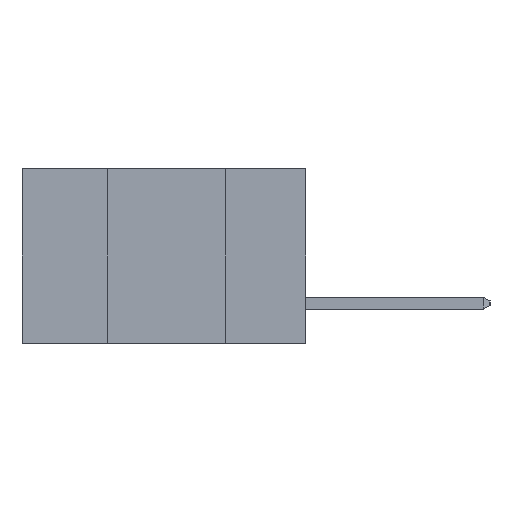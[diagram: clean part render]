
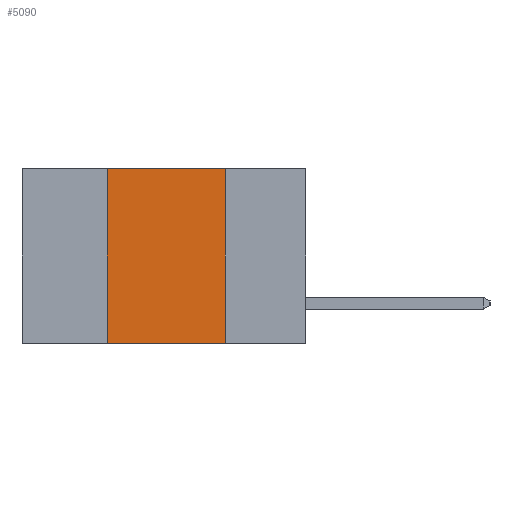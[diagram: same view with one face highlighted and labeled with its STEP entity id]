
A CAD part, left-side view. The second image highlights one B-rep face of the part: STEP entity #5090.
In plain terms, the highlighted planar face has unit normal (-1, 0, 0).
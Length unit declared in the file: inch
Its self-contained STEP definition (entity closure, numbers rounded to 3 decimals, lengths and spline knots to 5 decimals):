
#30 = EDGE_CURVE ( 'NONE', #3583, #1709, #10387, .T. ) ;
#32 = DIRECTION ( 'NONE',  ( 0., -1., 0. ) ) ;
#1709 = VERTEX_POINT ( 'NONE', #10174 ) ;
#1908 = EDGE_CURVE ( 'NONE', #9272, #1709, #5114, .T. ) ;
#2156 = DIRECTION ( 'NONE',  ( 0., 0., -1. ) ) ;
#2189 = ORIENTED_EDGE ( 'NONE', *, *, #1908, .T. ) ;
#2211 = VECTOR ( 'NONE', #10331, 39.37008 ) ;
#2306 = DIRECTION ( 'NONE',  ( 0., 0., -1. ) ) ;
#2318 = DIRECTION ( 'NONE',  ( 1., 0., 0. ) ) ;
#2360 = PLANE ( 'NONE',  #8290 ) ;
#2423 = CARTESIAN_POINT ( 'NONE',  ( 0., 0.6, 0. ) ) ;
#2826 = EDGE_CURVE ( 'NONE', #9272, #6959, #9616, .T. ) ;
#3561 = FACE_OUTER_BOUND ( 'NONE', #9331, .T. ) ;
#3583 = VERTEX_POINT ( 'NONE', #12828 ) ;
#3787 = ORIENTED_EDGE ( 'NONE', *, *, #6855, .F. ) ;
#5090 = ADVANCED_FACE ( 'NONE', ( #3561 ), #2360, .F. ) ;
#5114 = LINE ( 'NONE', #6919, #2211 ) ;
#6672 = VECTOR ( 'NONE', #9752, 39.37008 ) ;
#6855 = EDGE_CURVE ( 'NONE', #6959, #3583, #13334, .T. ) ;
#6919 = CARTESIAN_POINT ( 'NONE',  ( 0., 0.6, -0.37 ) ) ;
#6959 = VERTEX_POINT ( 'NONE', #7572 ) ;
#7572 = CARTESIAN_POINT ( 'NONE',  ( 0., 0.42, 0. ) ) ;
#8290 = AXIS2_PLACEMENT_3D ( 'NONE', #2423, #2318, #2306 ) ;
#8597 = ORIENTED_EDGE ( 'NONE', *, *, #30, .F. ) ;
#9272 = VERTEX_POINT ( 'NONE', #12992 ) ;
#9331 = EDGE_LOOP ( 'NONE', ( #8597, #3787, #10311, #2189 ) ) ;
#9616 = LINE ( 'NONE', #9888, #6672 ) ;
#9752 = DIRECTION ( 'NONE',  ( 0., 0., 1. ) ) ;
#9825 = CARTESIAN_POINT ( 'NONE',  ( 0., 0.17, 0. ) ) ;
#9888 = CARTESIAN_POINT ( 'NONE',  ( 0., 0.42, 0. ) ) ;
#10174 = CARTESIAN_POINT ( 'NONE',  ( 0., 0.17, -0.37 ) ) ;
#10311 = ORIENTED_EDGE ( 'NONE', *, *, #2826, .F. ) ;
#10331 = DIRECTION ( 'NONE',  ( 0., -1., 0. ) ) ;
#10387 = LINE ( 'NONE', #9825, #13231 ) ;
#10883 = CARTESIAN_POINT ( 'NONE',  ( 0., 0.6, 0. ) ) ;
#12331 = VECTOR ( 'NONE', #32, 39.37008 ) ;
#12828 = CARTESIAN_POINT ( 'NONE',  ( 0., 0.17, 0. ) ) ;
#12992 = CARTESIAN_POINT ( 'NONE',  ( 0., 0.42, -0.37 ) ) ;
#13231 = VECTOR ( 'NONE', #2156, 39.37008 ) ;
#13334 = LINE ( 'NONE', #10883, #12331 ) ;
